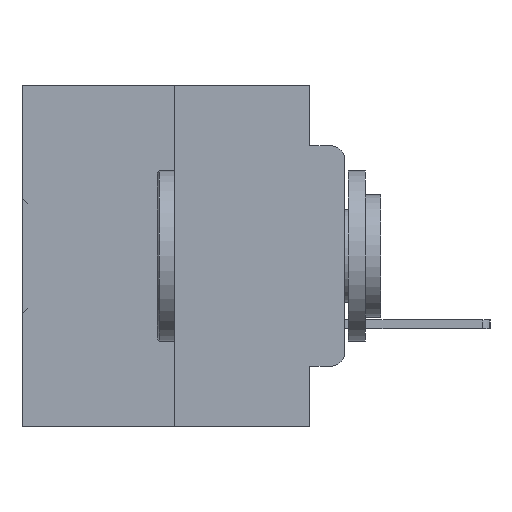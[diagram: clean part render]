
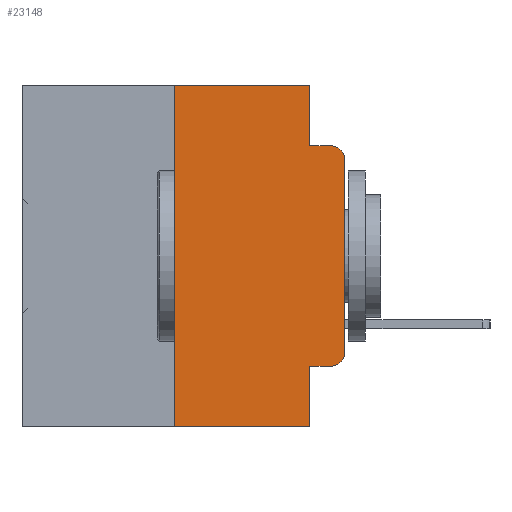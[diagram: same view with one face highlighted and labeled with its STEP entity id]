
A CAD part, left-side view. The second image highlights one B-rep face of the part: STEP entity #23148.
In plain terms, the highlighted planar face has unit normal (-1, 0, 0).
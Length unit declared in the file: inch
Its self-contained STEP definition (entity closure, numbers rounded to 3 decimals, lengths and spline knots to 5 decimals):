
#43 = VERTEX_POINT ( 'NONE', #31004 ) ;
#281 = VERTEX_POINT ( 'NONE', #31919 ) ;
#649 = CARTESIAN_POINT ( 'NONE',  ( 0., 0.25, 0. ) ) ;
#801 = ORIENTED_EDGE ( 'NONE', *, *, #3185, .F. ) ;
#932 = VERTEX_POINT ( 'NONE', #4409 ) ;
#1914 = CARTESIAN_POINT ( 'NONE',  ( 0., 0.25, 0. ) ) ;
#2051 = VERTEX_POINT ( 'NONE', #14555 ) ;
#3185 = EDGE_CURVE ( 'NONE', #26071, #6137, #9847, .T. ) ;
#3572 = CARTESIAN_POINT ( 'NONE',  ( 0., 0.051, 0. ) ) ;
#4408 = EDGE_CURVE ( 'NONE', #9828, #26071, #25899, .T. ) ;
#4409 = CARTESIAN_POINT ( 'NONE',  ( 0., 0., -0.3915 ) ) ;
#4740 = AXIS2_PLACEMENT_3D ( 'NONE', #6415, #9140, #27638 ) ;
#5225 = CARTESIAN_POINT ( 'NONE',  ( 0., 0.051, -0.0885 ) ) ;
#5237 = ORIENTED_EDGE ( 'NONE', *, *, #16696, .T. ) ;
#5573 = CARTESIAN_POINT ( 'NONE',  ( 0., 0.02, -0.0885 ) ) ;
#5846 = LINE ( 'NONE', #25688, #33148 ) ;
#6137 = VERTEX_POINT ( 'NONE', #5225 ) ;
#6415 = CARTESIAN_POINT ( 'NONE',  ( 0., 0.473, 0. ) ) ;
#6526 = ORIENTED_EDGE ( 'NONE', *, *, #12394, .T. ) ;
#6868 = EDGE_LOOP ( 'NONE', ( #20003, #6526, #14599, #801, #15449, #30132, #9930, #24860, #11653, #5237 ) ) ;
#7104 = DIRECTION ( 'NONE',  ( 0., 0., 1. ) ) ;
#7301 = CARTESIAN_POINT ( 'NONE',  ( 0., 0.051, -0.4115 ) ) ;
#7444 = VERTEX_POINT ( 'NONE', #13333 ) ;
#7872 = CARTESIAN_POINT ( 'NONE',  ( 0., 0.02, -0.1085 ) ) ;
#8733 = EDGE_CURVE ( 'NONE', #6137, #17336, #11133, .T. ) ;
#9051 = CARTESIAN_POINT ( 'NONE',  ( 0., 0., -0.1085 ) ) ;
#9140 = DIRECTION ( 'NONE',  ( 1., 0., 0. ) ) ;
#9828 = VERTEX_POINT ( 'NONE', #649 ) ;
#9847 = LINE ( 'NONE', #25361, #30058 ) ;
#9930 = ORIENTED_EDGE ( 'NONE', *, *, #27389, .T. ) ;
#10178 = CARTESIAN_POINT ( 'NONE',  ( 0., 0.473, -0.5 ) ) ;
#10589 = DIRECTION ( 'NONE',  ( 0., 0., -1. ) ) ;
#11082 = DIRECTION ( 'NONE',  ( -1., 0., 0. ) ) ;
#11133 = LINE ( 'NONE', #20254, #17490 ) ;
#11653 = ORIENTED_EDGE ( 'NONE', *, *, #21932, .T. ) ;
#12394 = EDGE_CURVE ( 'NONE', #32733, #17336, #32264, .T. ) ;
#13333 = CARTESIAN_POINT ( 'NONE',  ( 0., 0.051, -0.4115 ) ) ;
#14555 = CARTESIAN_POINT ( 'NONE',  ( 0., 0.051, -0.5 ) ) ;
#14599 = ORIENTED_EDGE ( 'NONE', *, *, #8733, .F. ) ;
#14766 = CARTESIAN_POINT ( 'NONE',  ( 0., 0.051, 0. ) ) ;
#15449 = ORIENTED_EDGE ( 'NONE', *, *, #4408, .F. ) ;
#16696 = EDGE_CURVE ( 'NONE', #281, #932, #23569, .T. ) ;
#17336 = VERTEX_POINT ( 'NONE', #5573 ) ;
#17490 = VECTOR ( 'NONE', #33294, 39.37008 ) ;
#17588 = FACE_OUTER_BOUND ( 'NONE', #6868, .T. ) ;
#17785 = AXIS2_PLACEMENT_3D ( 'NONE', #7872, #26416, #10589 ) ;
#19573 = EDGE_CURVE ( 'NONE', #932, #32733, #5846, .T. ) ;
#19591 = LINE ( 'NONE', #7301, #25657 ) ;
#19823 = DIRECTION ( 'NONE',  ( 0., 0., -1. ) ) ;
#19998 = CARTESIAN_POINT ( 'NONE',  ( 0., 0.473, 0. ) ) ;
#20003 = ORIENTED_EDGE ( 'NONE', *, *, #19573, .T. ) ;
#20254 = CARTESIAN_POINT ( 'NONE',  ( 0., 0.051, -0.0885 ) ) ;
#20549 = LINE ( 'NONE', #10178, #34327 ) ;
#20887 = DIRECTION ( 'NONE',  ( 0., 0., 1. ) ) ;
#21932 = EDGE_CURVE ( 'NONE', #7444, #281, #19591, .T. ) ;
#23148 = ADVANCED_FACE ( 'NONE', ( #17588 ), #25034, .F. ) ;
#23422 = LINE ( 'NONE', #3572, #28679 ) ;
#23569 = CIRCLE ( 'NONE', #27850, 0.02 ) ;
#24860 = ORIENTED_EDGE ( 'NONE', *, *, #27148, .F. ) ;
#25034 = PLANE ( 'NONE',  #4740 ) ;
#25084 = VECTOR ( 'NONE', #27678, 39.37008 ) ;
#25361 = CARTESIAN_POINT ( 'NONE',  ( 0., 0.051, 0. ) ) ;
#25391 = VECTOR ( 'NONE', #20887, 39.37008 ) ;
#25657 = VECTOR ( 'NONE', #28482, 39.37008 ) ;
#25688 = CARTESIAN_POINT ( 'NONE',  ( 0., 0., 0. ) ) ;
#25899 = LINE ( 'NONE', #19998, #25084 ) ;
#26071 = VERTEX_POINT ( 'NONE', #14766 ) ;
#26416 = DIRECTION ( 'NONE',  ( -1., 0., 0. ) ) ;
#26888 = CARTESIAN_POINT ( 'NONE',  ( 0., 0.02, -0.3915 ) ) ;
#27148 = EDGE_CURVE ( 'NONE', #7444, #2051, #23422, .T. ) ;
#27389 = EDGE_CURVE ( 'NONE', #43, #2051, #20549, .T. ) ;
#27638 = DIRECTION ( 'NONE',  ( 0., 0., -1. ) ) ;
#27678 = DIRECTION ( 'NONE',  ( 0., -1., 0. ) ) ;
#27850 = AXIS2_PLACEMENT_3D ( 'NONE', #26888, #11082, #29505 ) ;
#27969 = DIRECTION ( 'NONE',  ( 0., 0., -1. ) ) ;
#28482 = DIRECTION ( 'NONE',  ( 0., -1., 0. ) ) ;
#28625 = DIRECTION ( 'NONE',  ( 0., -1., 0. ) ) ;
#28679 = VECTOR ( 'NONE', #19823, 39.37008 ) ;
#29505 = DIRECTION ( 'NONE',  ( 0., 0., -1. ) ) ;
#30058 = VECTOR ( 'NONE', #27969, 39.37008 ) ;
#30132 = ORIENTED_EDGE ( 'NONE', *, *, #30616, .F. ) ;
#30616 = EDGE_CURVE ( 'NONE', #43, #9828, #32305, .T. ) ;
#31004 = CARTESIAN_POINT ( 'NONE',  ( 0., 0.25, -0.5 ) ) ;
#31919 = CARTESIAN_POINT ( 'NONE',  ( 0., 0.02, -0.4115 ) ) ;
#32264 = CIRCLE ( 'NONE', #17785, 0.02 ) ;
#32305 = LINE ( 'NONE', #1914, #25391 ) ;
#32733 = VERTEX_POINT ( 'NONE', #9051 ) ;
#33148 = VECTOR ( 'NONE', #7104, 39.37008 ) ;
#33294 = DIRECTION ( 'NONE',  ( 0., -1., 0. ) ) ;
#34327 = VECTOR ( 'NONE', #28625, 39.37008 ) ;
